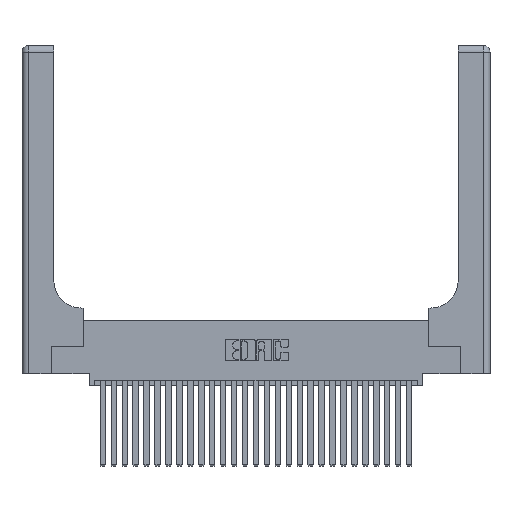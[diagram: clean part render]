
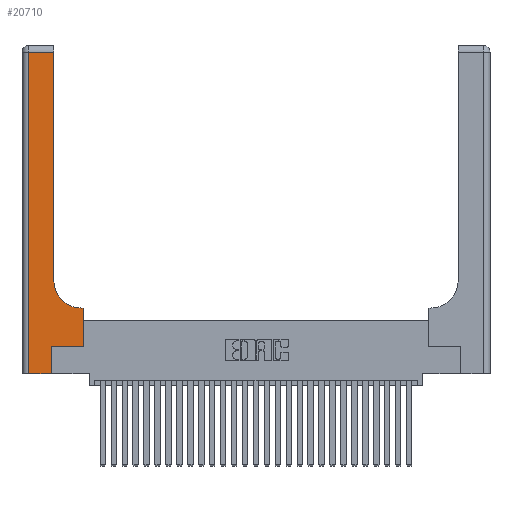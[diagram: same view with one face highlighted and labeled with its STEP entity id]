
A CAD part, top view. The second image highlights one B-rep face of the part: STEP entity #20710.
In plain terms, the highlighted planar face has unit normal (0, 0, 1).
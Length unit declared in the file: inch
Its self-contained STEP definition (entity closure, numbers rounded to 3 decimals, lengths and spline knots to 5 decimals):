
#175 = DIRECTION ( 'NONE',  ( 1., 0., 0. ) ) ;
#233 = VECTOR ( 'NONE', #7469, 39.37008 ) ;
#442 = EDGE_CURVE ( 'NONE', #4406, #16735, #11777, .T. ) ;
#897 = DIRECTION ( 'NONE',  ( 1., 0., 0. ) ) ;
#1272 = EDGE_LOOP ( 'NONE', ( #9396, #10870, #16930, #17670, #29611, #19099, #19811, #2104, #3565 ) ) ;
#1642 = CARTESIAN_POINT ( 'NONE',  ( 0.5585, 0.6, 0.37 ) ) ;
#2104 = ORIENTED_EDGE ( 'NONE', *, *, #2916, .T. ) ;
#2430 = CARTESIAN_POINT ( 'NONE',  ( 0., 0., 0.37 ) ) ;
#2519 = VECTOR ( 'NONE', #23477, 39.37008 ) ;
#2682 = CARTESIAN_POINT ( 'NONE',  ( 0.5585, 0.25, 0.37 ) ) ;
#2916 = EDGE_CURVE ( 'NONE', #11676, #7614, #8712, .T. ) ;
#3108 = VECTOR ( 'NONE', #16285, 39.37008 ) ;
#3132 = LINE ( 'NONE', #26647, #14739 ) ;
#3565 = ORIENTED_EDGE ( 'NONE', *, *, #27001, .T. ) ;
#4128 = VECTOR ( 'NONE', #9505, 39.37008 ) ;
#4406 = VERTEX_POINT ( 'NONE', #13294 ) ;
#4630 = CARTESIAN_POINT ( 'NONE',  ( 0.06, 0., 0.37 ) ) ;
#4799 = CARTESIAN_POINT ( 'NONE',  ( 0.269, 0.25, 0.37 ) ) ;
#5148 = CARTESIAN_POINT ( 'NONE',  ( 0.06, 3., 0.37 ) ) ;
#5929 = EDGE_CURVE ( 'NONE', #27452, #9504, #20363, .T. ) ;
#7098 = CARTESIAN_POINT ( 'NONE',  ( 0., 3., 0.37 ) ) ;
#7233 = VERTEX_POINT ( 'NONE', #4630 ) ;
#7469 = DIRECTION ( 'NONE',  ( 0., -1., 0. ) ) ;
#7596 = LINE ( 'NONE', #27343, #19132 ) ;
#7614 = VERTEX_POINT ( 'NONE', #27292 ) ;
#8068 = CARTESIAN_POINT ( 'NONE',  ( 0.269, 0., 0.37 ) ) ;
#8712 = LINE ( 'NONE', #27978, #2519 ) ;
#8958 = CARTESIAN_POINT ( 'NONE',  ( 0.2915, 0.85, 0.37 ) ) ;
#9155 = DIRECTION ( 'NONE',  ( 0., 1., 0. ) ) ;
#9396 = ORIENTED_EDGE ( 'NONE', *, *, #13159, .T. ) ;
#9504 = VERTEX_POINT ( 'NONE', #2682 ) ;
#9505 = DIRECTION ( 'NONE',  ( 0., 1., 0. ) ) ;
#10335 = LINE ( 'NONE', #20919, #4128 ) ;
#10870 = ORIENTED_EDGE ( 'NONE', *, *, #442, .T. ) ;
#10888 = EDGE_CURVE ( 'NONE', #26390, #27452, #3132, .T. ) ;
#11676 = VERTEX_POINT ( 'NONE', #1642 ) ;
#11772 = DIRECTION ( 'NONE',  ( -1., 0., 0. ) ) ;
#11777 = LINE ( 'NONE', #20300, #29125 ) ;
#12017 = CARTESIAN_POINT ( 'NONE',  ( 0.06, 2.94, 0.37 ) ) ;
#12465 = FACE_OUTER_BOUND ( 'NONE', #1272, .T. ) ;
#13159 = EDGE_CURVE ( 'NONE', #14951, #4406, #7596, .T. ) ;
#13294 = CARTESIAN_POINT ( 'NONE',  ( 0.2915, 2.94, 0.37 ) ) ;
#13915 = EDGE_CURVE ( 'NONE', #16735, #7233, #18727, .T. ) ;
#14739 = VECTOR ( 'NONE', #19970, 39.37008 ) ;
#14809 = DIRECTION ( 'NONE',  ( 0., 0., -1. ) ) ;
#14951 = VERTEX_POINT ( 'NONE', #8958 ) ;
#16285 = DIRECTION ( 'NONE',  ( 1., 0., 0. ) ) ;
#16735 = VERTEX_POINT ( 'NONE', #12017 ) ;
#16930 = ORIENTED_EDGE ( 'NONE', *, *, #13915, .T. ) ;
#17552 = CIRCLE ( 'NONE', #18718, 0.25 ) ;
#17670 = ORIENTED_EDGE ( 'NONE', *, *, #25526, .T. ) ;
#18718 = AXIS2_PLACEMENT_3D ( 'NONE', #28345, #14809, #897 ) ;
#18727 = LINE ( 'NONE', #5148, #233 ) ;
#19099 = ORIENTED_EDGE ( 'NONE', *, *, #5929, .T. ) ;
#19132 = VECTOR ( 'NONE', #9155, 39.37008 ) ;
#19745 = CARTESIAN_POINT ( 'NONE',  ( 0.269, 0.25, 0.37 ) ) ;
#19811 = ORIENTED_EDGE ( 'NONE', *, *, #27766, .T. ) ;
#19970 = DIRECTION ( 'NONE',  ( 0., 1., 0. ) ) ;
#20114 = DIRECTION ( 'NONE',  ( -1., 0., 0. ) ) ;
#20300 = CARTESIAN_POINT ( 'NONE',  ( 0., 2.94, 0.37 ) ) ;
#20363 = LINE ( 'NONE', #4799, #25613 ) ;
#20710 = ADVANCED_FACE ( 'NONE', ( #12465 ), #23123, .F. ) ;
#20919 = CARTESIAN_POINT ( 'NONE',  ( 0.5585, 0.25, 0.37 ) ) ;
#23123 = PLANE ( 'NONE',  #23898 ) ;
#23477 = DIRECTION ( 'NONE',  ( -1., 0., 0. ) ) ;
#23898 = AXIS2_PLACEMENT_3D ( 'NONE', #7098, #25371, #11772 ) ;
#25371 = DIRECTION ( 'NONE',  ( 0., 0., -1. ) ) ;
#25526 = EDGE_CURVE ( 'NONE', #7233, #26390, #26767, .T. ) ;
#25613 = VECTOR ( 'NONE', #175, 39.37008 ) ;
#26390 = VERTEX_POINT ( 'NONE', #8068 ) ;
#26647 = CARTESIAN_POINT ( 'NONE',  ( 0.269, 0., 0.37 ) ) ;
#26767 = LINE ( 'NONE', #2430, #3108 ) ;
#27001 = EDGE_CURVE ( 'NONE', #7614, #14951, #17552, .T. ) ;
#27292 = CARTESIAN_POINT ( 'NONE',  ( 0.5415, 0.6, 0.37 ) ) ;
#27343 = CARTESIAN_POINT ( 'NONE',  ( 0.2915, 3., 0.37 ) ) ;
#27452 = VERTEX_POINT ( 'NONE', #19745 ) ;
#27766 = EDGE_CURVE ( 'NONE', #9504, #11676, #10335, .T. ) ;
#27978 = CARTESIAN_POINT ( 'NONE',  ( 0.2915, 0.6, 0.37 ) ) ;
#28345 = CARTESIAN_POINT ( 'NONE',  ( 0.5415, 0.85, 0.37 ) ) ;
#29125 = VECTOR ( 'NONE', #20114, 39.37008 ) ;
#29611 = ORIENTED_EDGE ( 'NONE', *, *, #10888, .T. ) ;
